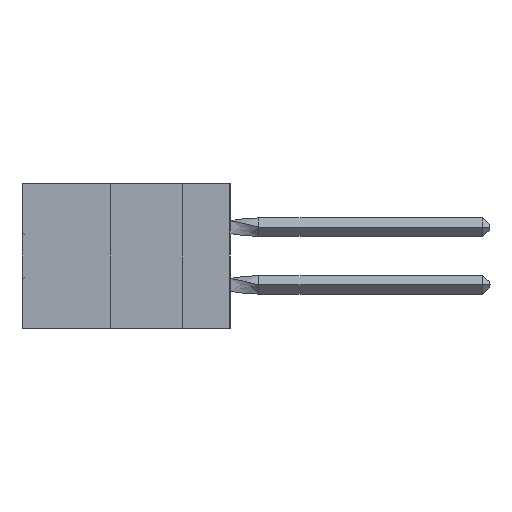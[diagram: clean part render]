
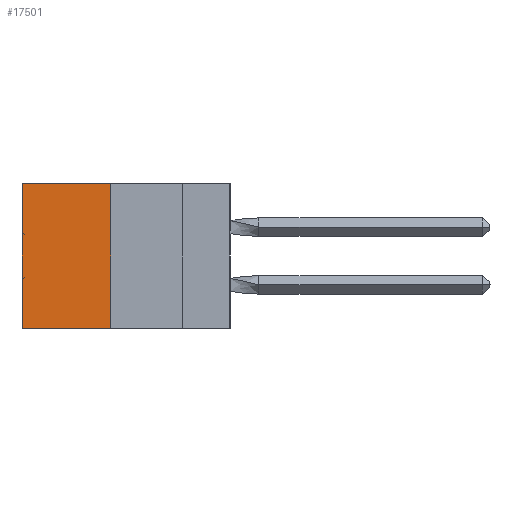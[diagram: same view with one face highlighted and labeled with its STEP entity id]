
A CAD part, left-side view. The second image highlights one B-rep face of the part: STEP entity #17501.
In plain terms, the highlighted planar face has unit normal (-1, 0, 0).
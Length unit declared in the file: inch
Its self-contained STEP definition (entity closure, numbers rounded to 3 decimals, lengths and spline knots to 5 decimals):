
#4567 = PLANE ( 'NONE',  #12224 ) ;
#6066 = VERTEX_POINT ( 'NONE', #20233 ) ;
#6541 = ORIENTED_EDGE ( 'NONE', *, *, #9079, .T. ) ;
#7085 = ORIENTED_EDGE ( 'NONE', *, *, #47563, .F. ) ;
#7452 = CARTESIAN_POINT ( 'NONE',  ( 0.305, 0.413, -0.5 ) ) ;
#9079 = EDGE_CURVE ( 'NONE', #42284, #39397, #47429, .T. ) ;
#10847 = ORIENTED_EDGE ( 'NONE', *, *, #37171, .T. ) ;
#12224 = AXIS2_PLACEMENT_3D ( 'NONE', #56468, #39606, #13397 ) ;
#13397 = DIRECTION ( 'NONE',  ( 0., 0., -1. ) ) ;
#14908 = FACE_OUTER_BOUND ( 'NONE', #18595, .T. ) ;
#16220 = DIRECTION ( 'NONE',  ( 0., 1., 0. ) ) ;
#17441 = DIRECTION ( 'NONE',  ( 0., 0., -1. ) ) ;
#17501 = ADVANCED_FACE ( 'NONE', ( #14908 ), #4567, .F. ) ;
#18595 = EDGE_LOOP ( 'NONE', ( #6541, #7085, #43445, #10847 ) ) ;
#20233 = CARTESIAN_POINT ( 'NONE',  ( 0.305, 0.413, -0.5 ) ) ;
#20929 = CARTESIAN_POINT ( 'NONE',  ( 0.305, 0.413, -0.5 ) ) ;
#22755 = LINE ( 'NONE', #7452, #53531 ) ;
#24027 = CARTESIAN_POINT ( 'NONE',  ( 0.305, 0.413, 0. ) ) ;
#26558 = LINE ( 'NONE', #55452, #27292 ) ;
#27292 = VECTOR ( 'NONE', #16220, 39.37008 ) ;
#29118 = DIRECTION ( 'NONE',  ( 0., 1., 0. ) ) ;
#29169 = DIRECTION ( 'NONE',  ( 0., 0., -1. ) ) ;
#34196 = CARTESIAN_POINT ( 'NONE',  ( 0.305, 0.72, -0.5 ) ) ;
#34359 = CARTESIAN_POINT ( 'NONE',  ( 0.305, 0.72, -0.5 ) ) ;
#35624 = CARTESIAN_POINT ( 'NONE',  ( 0.305, 0.72, 0. ) ) ;
#35775 = VECTOR ( 'NONE', #17441, 39.37008 ) ;
#37171 = EDGE_CURVE ( 'NONE', #37722, #42284, #26558, .T. ) ;
#37722 = VERTEX_POINT ( 'NONE', #24027 ) ;
#37819 = EDGE_CURVE ( 'NONE', #37722, #6066, #50370, .T. ) ;
#39397 = VERTEX_POINT ( 'NONE', #34359 ) ;
#39606 = DIRECTION ( 'NONE',  ( 1., 0., 0. ) ) ;
#42284 = VERTEX_POINT ( 'NONE', #35624 ) ;
#43445 = ORIENTED_EDGE ( 'NONE', *, *, #37819, .F. ) ;
#47429 = LINE ( 'NONE', #34196, #35775 ) ;
#47563 = EDGE_CURVE ( 'NONE', #6066, #39397, #22755, .T. ) ;
#50370 = LINE ( 'NONE', #20929, #56572 ) ;
#53531 = VECTOR ( 'NONE', #29118, 39.37008 ) ;
#55452 = CARTESIAN_POINT ( 'NONE',  ( 0.305, 0.413, 0. ) ) ;
#56468 = CARTESIAN_POINT ( 'NONE',  ( 0.305, 0.413, -0.5 ) ) ;
#56572 = VECTOR ( 'NONE', #29169, 39.37008 ) ;
